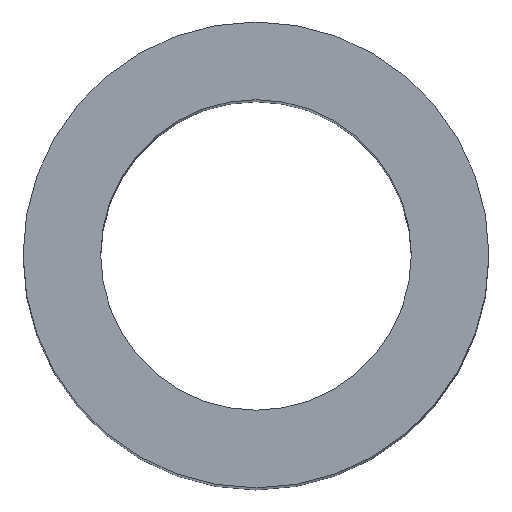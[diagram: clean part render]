
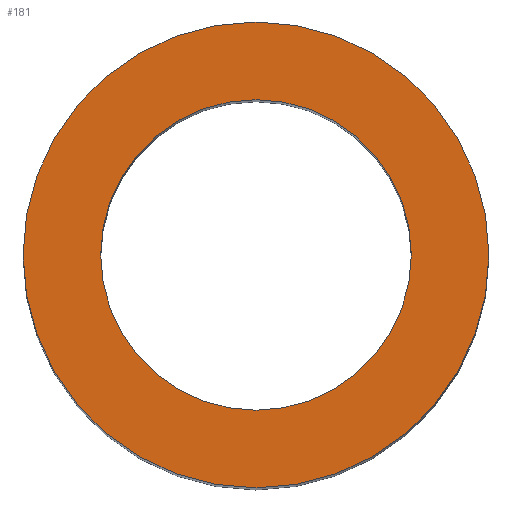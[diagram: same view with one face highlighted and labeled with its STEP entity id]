
A CAD part, top view. The second image highlights one B-rep face of the part: STEP entity #181.
In plain terms, the highlighted planar face has unit normal (0, 0, 1).
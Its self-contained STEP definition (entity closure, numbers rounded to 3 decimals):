
#2 = DIRECTION ( 'NONE',  ( 0., 0., 1. ) ) ;
#5 = CARTESIAN_POINT ( 'NONE',  ( -2.032, 0., 16.002 ) ) ;
#15 = VERTEX_POINT ( 'NONE', #151 ) ;
#17 = EDGE_LOOP ( 'NONE', ( #161, #121 ) ) ;
#21 = DIRECTION ( 'NONE',  ( 1., 0., 0. ) ) ;
#23 = CARTESIAN_POINT ( 'NONE',  ( 0., 0., 16.002 ) ) ;
#26 = DIRECTION ( 'NONE',  ( 1., 0., 0. ) ) ;
#27 = DIRECTION ( 'NONE',  ( 0., 0., 1. ) ) ;
#28 = PLANE ( 'NONE',  #74 ) ;
#29 = DIRECTION ( 'NONE',  ( 1., 0., 0. ) ) ;
#30 = DIRECTION ( 'NONE',  ( 1., 0., 0. ) ) ;
#34 = CARTESIAN_POINT ( 'NONE',  ( 0., 0., 16.002 ) ) ;
#56 = CARTESIAN_POINT ( 'NONE',  ( 0., 0., 16.002 ) ) ;
#74 = AXIS2_PLACEMENT_3D ( 'NONE', #34, #27, #21 ) ;
#80 = AXIS2_PLACEMENT_3D ( 'NONE', #153, #119, #118 ) ;
#85 = AXIS2_PLACEMENT_3D ( 'NONE', #86, #115, #26 ) ;
#86 = CARTESIAN_POINT ( 'NONE',  ( 0., 0., 16.002 ) ) ;
#91 = ORIENTED_EDGE ( 'NONE', *, *, #124, .T. ) ;
#93 = EDGE_CURVE ( 'NONE', #15, #197, #155, .T. ) ;
#94 = AXIS2_PLACEMENT_3D ( 'NONE', #23, #109, #29 ) ;
#99 = AXIS2_PLACEMENT_3D ( 'NONE', #56, #2, #30 ) ;
#108 = FACE_OUTER_BOUND ( 'NONE', #167, .T. ) ;
#109 = DIRECTION ( 'NONE',  ( 0., 0., 1. ) ) ;
#115 = DIRECTION ( 'NONE',  ( 0., 0., 1. ) ) ;
#118 = DIRECTION ( 'NONE',  ( 1., 0., 0. ) ) ;
#119 = DIRECTION ( 'NONE',  ( 0., 0., 1. ) ) ;
#121 = ORIENTED_EDGE ( 'NONE', *, *, #157, .F. ) ;
#124 = EDGE_CURVE ( 'NONE', #197, #15, #148, .T. ) ;
#131 = FACE_BOUND ( 'NONE', #17, .T. ) ;
#141 = CIRCLE ( 'NONE', #85, 2.032 ) ;
#143 = EDGE_CURVE ( 'NONE', #179, #189, #141, .T. ) ;
#144 = CIRCLE ( 'NONE', #80, 2.032 ) ;
#148 = CIRCLE ( 'NONE', #94, 3.048 ) ;
#151 = CARTESIAN_POINT ( 'NONE',  ( -3.048, 0., 16.002 ) ) ;
#153 = CARTESIAN_POINT ( 'NONE',  ( 0., 0., 16.002 ) ) ;
#155 = CIRCLE ( 'NONE', #99, 3.048 ) ;
#157 = EDGE_CURVE ( 'NONE', #189, #179, #144, .T. ) ;
#161 = ORIENTED_EDGE ( 'NONE', *, *, #143, .F. ) ;
#167 = EDGE_LOOP ( 'NONE', ( #184, #91 ) ) ;
#179 = VERTEX_POINT ( 'NONE', #5 ) ;
#181 = ADVANCED_FACE ( 'NONE', ( #131, #108 ), #28, .T. ) ;
#184 = ORIENTED_EDGE ( 'NONE', *, *, #93, .T. ) ;
#185 = CARTESIAN_POINT ( 'NONE',  ( 2.032, 0., 16.002 ) ) ;
#189 = VERTEX_POINT ( 'NONE', #185 ) ;
#190 = CARTESIAN_POINT ( 'NONE',  ( 3.048, 0., 16.002 ) ) ;
#197 = VERTEX_POINT ( 'NONE', #190 ) ;
